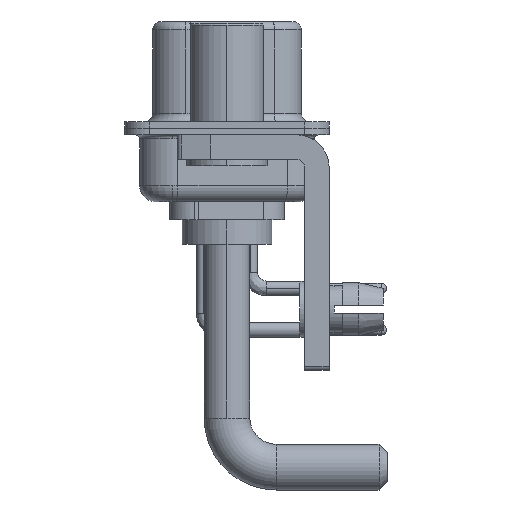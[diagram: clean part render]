
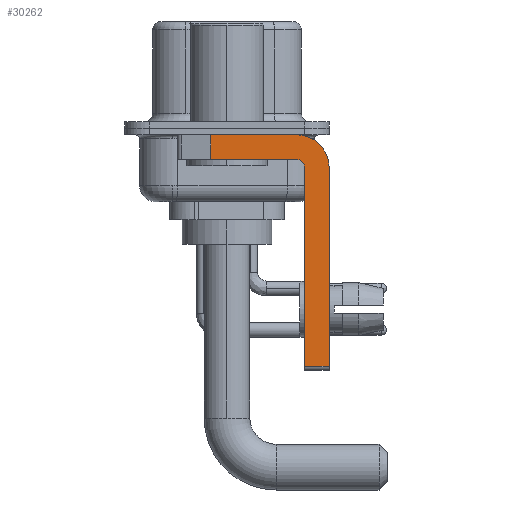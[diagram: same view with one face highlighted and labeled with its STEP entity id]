
A CAD part, left-side view. The second image highlights one B-rep face of the part: STEP entity #30262.
In plain terms, the highlighted planar face has unit normal (-1, 0, 0).
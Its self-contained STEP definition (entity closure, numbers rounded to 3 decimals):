
#337 = EDGE_CURVE ( 'NONE', #8761, #4472, #30109, .T. ) ;
#366 = LINE ( 'NONE', #5229, #19176 ) ;
#612 = DIRECTION ( 'NONE',  ( 0., 0., -1. ) ) ;
#651 = CARTESIAN_POINT ( 'NONE',  ( -2.9, -4.25, -1.9 ) ) ;
#1192 = ORIENTED_EDGE ( 'NONE', *, *, #337, .F. ) ;
#2826 = EDGE_CURVE ( 'NONE', #4822, #4114, #366, .T. ) ;
#3273 = ORIENTED_EDGE ( 'NONE', *, *, #27660, .F. ) ;
#3871 = EDGE_CURVE ( 'NONE', #18759, #15040, #10811, .T. ) ;
#4069 = VECTOR ( 'NONE', #612, 1000. ) ;
#4114 = VERTEX_POINT ( 'NONE', #29842 ) ;
#4472 = VERTEX_POINT ( 'NONE', #26220 ) ;
#4822 = VERTEX_POINT ( 'NONE', #16727 ) ;
#5085 = LINE ( 'NONE', #26835, #30147 ) ;
#5229 = CARTESIAN_POINT ( 'NONE',  ( -2.9, 3., -0.4 ) ) ;
#5655 = DIRECTION ( 'NONE',  ( 0., 0., 1. ) ) ;
#5868 = VERTEX_POINT ( 'NONE', #14370 ) ;
#6974 = CARTESIAN_POINT ( 'NONE',  ( -2.9, -4.25, -2.4 ) ) ;
#7294 = ORIENTED_EDGE ( 'NONE', *, *, #19883, .F. ) ;
#7615 = ORIENTED_EDGE ( 'NONE', *, *, #17602, .T. ) ;
#7692 = ORIENTED_EDGE ( 'NONE', *, *, #17886, .T. ) ;
#8065 = CARTESIAN_POINT ( 'NONE',  ( -2.9, -6.25, -2.4 ) ) ;
#8343 = DIRECTION ( 'NONE',  ( 0., 0., -1. ) ) ;
#8411 = AXIS2_PLACEMENT_3D ( 'NONE', #27564, #29986, #5655 ) ;
#8761 = VERTEX_POINT ( 'NONE', #651 ) ;
#8810 = LINE ( 'NONE', #18418, #14224 ) ;
#9869 = FACE_OUTER_BOUND ( 'NONE', #30762, .T. ) ;
#10491 = CIRCLE ( 'NONE', #8411, 0.5 ) ;
#10811 = LINE ( 'NONE', #8065, #4069 ) ;
#10846 = ORIENTED_EDGE ( 'NONE', *, *, #3871, .F. ) ;
#12465 = DIRECTION ( 'NONE',  ( 1., 0., 0. ) ) ;
#13232 = DIRECTION ( 'NONE',  ( 1., 0., 0. ) ) ;
#14224 = VECTOR ( 'NONE', #14499, 1000. ) ;
#14370 = CARTESIAN_POINT ( 'NONE',  ( -2.9, -4.75, -14.55 ) ) ;
#14499 = DIRECTION ( 'NONE',  ( 0., 0., 1. ) ) ;
#14981 = DIRECTION ( 'NONE',  ( 0., 0., -1. ) ) ;
#15040 = VERTEX_POINT ( 'NONE', #15573 ) ;
#15302 = DIRECTION ( 'NONE',  ( 0., -1., 0. ) ) ;
#15563 = EDGE_CURVE ( 'NONE', #5868, #21912, #8810, .T. ) ;
#15573 = CARTESIAN_POINT ( 'NONE',  ( -2.9, -6.25, -14.55 ) ) ;
#16727 = CARTESIAN_POINT ( 'NONE',  ( -2.9, 0.978, -0.4 ) ) ;
#17359 = DIRECTION ( 'NONE',  ( 0., 0., -1. ) ) ;
#17602 = EDGE_CURVE ( 'NONE', #4822, #4472, #5085, .T. ) ;
#17886 = EDGE_CURVE ( 'NONE', #5868, #15040, #20980, .T. ) ;
#18136 = AXIS2_PLACEMENT_3D ( 'NONE', #6974, #12465, #17359 ) ;
#18418 = CARTESIAN_POINT ( 'NONE',  ( -2.9, -4.75, -14.8 ) ) ;
#18759 = VERTEX_POINT ( 'NONE', #27163 ) ;
#19176 = VECTOR ( 'NONE', #15302, 1000. ) ;
#19607 = AXIS2_PLACEMENT_3D ( 'NONE', #30265, #13232, #8343 ) ;
#19788 = PLANE ( 'NONE',  #18136 ) ;
#19883 = EDGE_CURVE ( 'NONE', #21912, #8761, #10491, .T. ) ;
#20980 = LINE ( 'NONE', #26009, #31110 ) ;
#21912 = VERTEX_POINT ( 'NONE', #23183 ) ;
#23183 = CARTESIAN_POINT ( 'NONE',  ( -2.9, -4.75, -2.4 ) ) ;
#24662 = DIRECTION ( 'NONE',  ( 0., -1., 0. ) ) ;
#24945 = CARTESIAN_POINT ( 'NONE',  ( -2.9, -4.25, -1.9 ) ) ;
#25321 = CIRCLE ( 'NONE', #19607, 2. ) ;
#26009 = CARTESIAN_POINT ( 'NONE',  ( -2.9, -4.25, -14.55 ) ) ;
#26220 = CARTESIAN_POINT ( 'NONE',  ( -2.9, 0.978, -1.9 ) ) ;
#26462 = ORIENTED_EDGE ( 'NONE', *, *, #15563, .F. ) ;
#26835 = CARTESIAN_POINT ( 'NONE',  ( -2.9, 0.978, -1.9 ) ) ;
#27163 = CARTESIAN_POINT ( 'NONE',  ( -2.9, -6.25, -2.4 ) ) ;
#27564 = CARTESIAN_POINT ( 'NONE',  ( -2.9, -4.25, -2.4 ) ) ;
#27660 = EDGE_CURVE ( 'NONE', #4114, #18759, #25321, .T. ) ;
#27683 = DIRECTION ( 'NONE',  ( 0., 1., 0. ) ) ;
#28368 = ORIENTED_EDGE ( 'NONE', *, *, #2826, .F. ) ;
#29842 = CARTESIAN_POINT ( 'NONE',  ( -2.9, -4.25, -0.4 ) ) ;
#29986 = DIRECTION ( 'NONE',  ( -1., 0., 0. ) ) ;
#30109 = LINE ( 'NONE', #24945, #31405 ) ;
#30147 = VECTOR ( 'NONE', #14981, 1000. ) ;
#30262 = ADVANCED_FACE ( 'NONE', ( #9869 ), #19788, .F. ) ;
#30265 = CARTESIAN_POINT ( 'NONE',  ( -2.9, -4.25, -2.4 ) ) ;
#30762 = EDGE_LOOP ( 'NONE', ( #28368, #7615, #1192, #7294, #26462, #7692, #10846, #3273 ) ) ;
#31110 = VECTOR ( 'NONE', #24662, 1000. ) ;
#31405 = VECTOR ( 'NONE', #27683, 1000. ) ;
